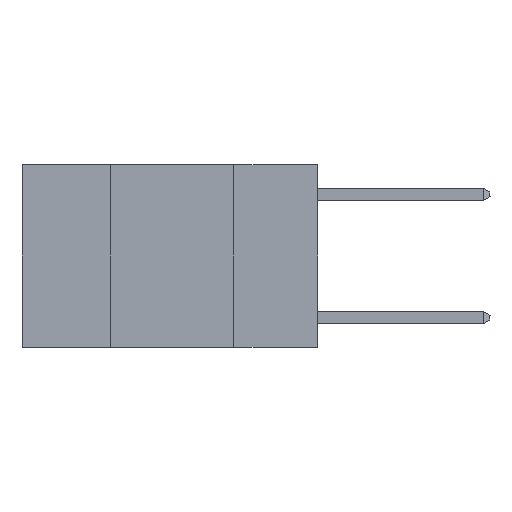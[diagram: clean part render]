
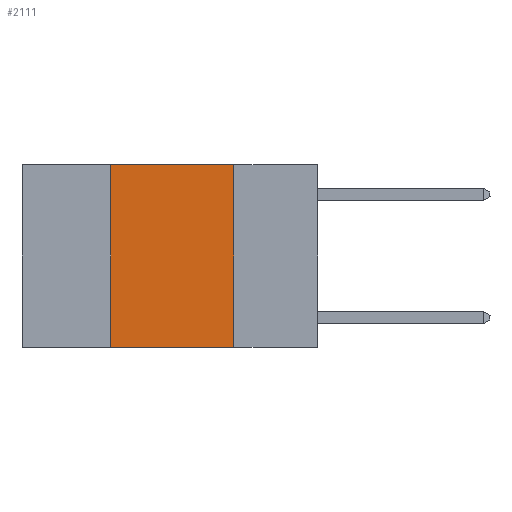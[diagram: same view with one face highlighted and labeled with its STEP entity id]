
A CAD part, left-side view. The second image highlights one B-rep face of the part: STEP entity #2111.
In plain terms, the highlighted planar face has unit normal (-1, 0, 0).
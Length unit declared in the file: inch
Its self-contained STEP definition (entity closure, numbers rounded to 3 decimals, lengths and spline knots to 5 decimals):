
#51 = DIRECTION ( 'NONE',  ( 0., -1., 0. ) ) ;
#68 = DIRECTION ( 'NONE',  ( 0., 0., 1. ) ) ;
#144 = DIRECTION ( 'NONE',  ( 0., 0., -1. ) ) ;
#418 = EDGE_CURVE ( 'NONE', #2692, #1544, #4443, .T. ) ;
#706 = CARTESIAN_POINT ( 'NONE',  ( 0., 0.17, 0. ) ) ;
#733 = LINE ( 'NONE', #9331, #2511 ) ;
#918 = FACE_OUTER_BOUND ( 'NONE', #9132, .T. ) ;
#1099 = EDGE_CURVE ( 'NONE', #2692, #3612, #733, .T. ) ;
#1266 = AXIS2_PLACEMENT_3D ( 'NONE', #8617, #6077, #144 ) ;
#1337 = CARTESIAN_POINT ( 'NONE',  ( 0., 0.17, 0. ) ) ;
#1544 = VERTEX_POINT ( 'NONE', #6603 ) ;
#2111 = ADVANCED_FACE ( 'NONE', ( #918 ), #5217, .F. ) ;
#2121 = CARTESIAN_POINT ( 'NONE',  ( 0., 0.42, 0. ) ) ;
#2475 = LINE ( 'NONE', #706, #9809 ) ;
#2511 = VECTOR ( 'NONE', #68, 39.37008 ) ;
#2692 = VERTEX_POINT ( 'NONE', #8979 ) ;
#3612 = VERTEX_POINT ( 'NONE', #2121 ) ;
#4236 = DIRECTION ( 'NONE',  ( 0., -1., 0. ) ) ;
#4443 = LINE ( 'NONE', #10246, #5810 ) ;
#4517 = EDGE_CURVE ( 'NONE', #3612, #7977, #5712, .T. ) ;
#5217 = PLANE ( 'NONE',  #1266 ) ;
#5507 = ORIENTED_EDGE ( 'NONE', *, *, #7629, .F. ) ;
#5712 = LINE ( 'NONE', #9248, #10314 ) ;
#5810 = VECTOR ( 'NONE', #4236, 39.37008 ) ;
#6077 = DIRECTION ( 'NONE',  ( 1., 0., 0. ) ) ;
#6603 = CARTESIAN_POINT ( 'NONE',  ( 0., 0.17, -0.37 ) ) ;
#7629 = EDGE_CURVE ( 'NONE', #7977, #1544, #2475, .T. ) ;
#7894 = ORIENTED_EDGE ( 'NONE', *, *, #4517, .F. ) ;
#7977 = VERTEX_POINT ( 'NONE', #1337 ) ;
#8389 = ORIENTED_EDGE ( 'NONE', *, *, #418, .T. ) ;
#8617 = CARTESIAN_POINT ( 'NONE',  ( 0., 0.6, 0. ) ) ;
#8653 = ORIENTED_EDGE ( 'NONE', *, *, #1099, .F. ) ;
#8979 = CARTESIAN_POINT ( 'NONE',  ( 0., 0.42, -0.37 ) ) ;
#9132 = EDGE_LOOP ( 'NONE', ( #5507, #7894, #8653, #8389 ) ) ;
#9186 = DIRECTION ( 'NONE',  ( 0., 0., -1. ) ) ;
#9248 = CARTESIAN_POINT ( 'NONE',  ( 0., 0.6, 0. ) ) ;
#9331 = CARTESIAN_POINT ( 'NONE',  ( 0., 0.42, 0. ) ) ;
#9809 = VECTOR ( 'NONE', #9186, 39.37008 ) ;
#10246 = CARTESIAN_POINT ( 'NONE',  ( 0., 0.6, -0.37 ) ) ;
#10314 = VECTOR ( 'NONE', #51, 39.37008 ) ;
